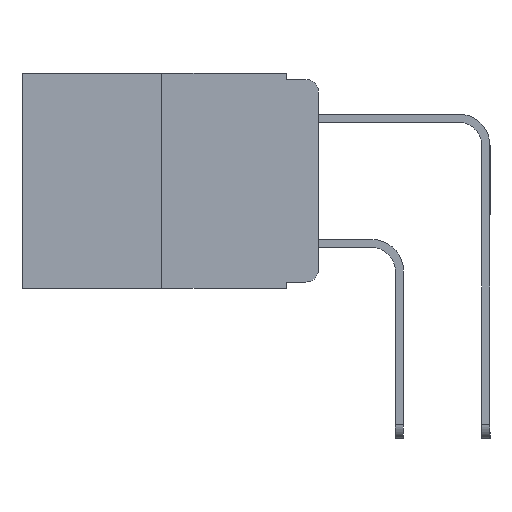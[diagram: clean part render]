
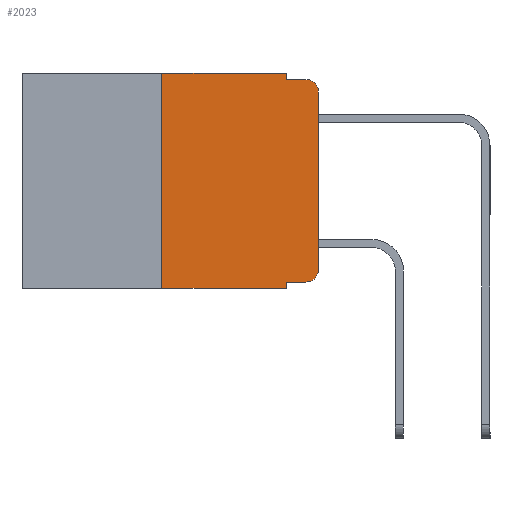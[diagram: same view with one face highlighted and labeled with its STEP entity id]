
A CAD part, left-side view. The second image highlights one B-rep face of the part: STEP entity #2023.
In plain terms, the highlighted planar face has unit normal (-1, 0, 0).
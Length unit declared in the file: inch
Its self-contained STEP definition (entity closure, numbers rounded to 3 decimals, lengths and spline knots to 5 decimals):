
#617 = LINE ( 'NONE', #1569, #8385 ) ;
#665 = LINE ( 'NONE', #15639, #1189 ) ;
#991 = ORIENTED_EDGE ( 'NONE', *, *, #13406, .F. ) ;
#1111 = VERTEX_POINT ( 'NONE', #16406 ) ;
#1169 = EDGE_CURVE ( 'NONE', #15016, #19149, #10449, .T. ) ;
#1189 = VECTOR ( 'NONE', #4652, 39.37008 ) ;
#1569 = CARTESIAN_POINT ( 'NONE',  ( 0., 0.25, 0. ) ) ;
#2023 = ADVANCED_FACE ( 'NONE', ( #3093 ), #8099, .F. ) ;
#2082 = VERTEX_POINT ( 'NONE', #9774 ) ;
#2101 = DIRECTION ( 'NONE',  ( 0., 0., -1. ) ) ;
#2270 = EDGE_CURVE ( 'NONE', #2365, #15016, #18591, .T. ) ;
#2335 = DIRECTION ( 'NONE',  ( -1., 0., 0. ) ) ;
#2365 = VERTEX_POINT ( 'NONE', #5889 ) ;
#3093 = FACE_OUTER_BOUND ( 'NONE', #9705, .T. ) ;
#3353 = ORIENTED_EDGE ( 'NONE', *, *, #5656, .F. ) ;
#3389 = EDGE_CURVE ( 'NONE', #2365, #6398, #12743, .T. ) ;
#3674 = LINE ( 'NONE', #16158, #15785 ) ;
#3875 = LINE ( 'NONE', #20039, #4422 ) ;
#3889 = CARTESIAN_POINT ( 'NONE',  ( 0., 0.051, -0.333 ) ) ;
#4422 = VECTOR ( 'NONE', #9297, 39.37008 ) ;
#4532 = EDGE_CURVE ( 'NONE', #1111, #14957, #617, .T. ) ;
#4652 = DIRECTION ( 'NONE',  ( 0., 0., -1. ) ) ;
#4967 = DIRECTION ( 'NONE',  ( -1., 0., 0. ) ) ;
#5305 = DIRECTION ( 'NONE',  ( 0., -1., 0. ) ) ;
#5582 = CARTESIAN_POINT ( 'NONE',  ( 0., 0.25, 0. ) ) ;
#5656 = EDGE_CURVE ( 'NONE', #16372, #13389, #665, .T. ) ;
#5866 = VERTEX_POINT ( 'NONE', #16166 ) ;
#5889 = CARTESIAN_POINT ( 'NONE',  ( 0., 0.051, -0.333 ) ) ;
#6398 = VERTEX_POINT ( 'NONE', #12817 ) ;
#6485 = CARTESIAN_POINT ( 'NONE',  ( 0., 0.473, 0. ) ) ;
#6742 = VECTOR ( 'NONE', #13379, 39.37008 ) ;
#7048 = ORIENTED_EDGE ( 'NONE', *, *, #2270, .T. ) ;
#7131 = ORIENTED_EDGE ( 'NONE', *, *, #9900, .T. ) ;
#7267 = ORIENTED_EDGE ( 'NONE', *, *, #18051, .T. ) ;
#7844 = EDGE_CURVE ( 'NONE', #13389, #5866, #14094, .T. ) ;
#7992 = CARTESIAN_POINT ( 'NONE',  ( 0., 0.473, -0.343 ) ) ;
#8065 = ORIENTED_EDGE ( 'NONE', *, *, #4532, .F. ) ;
#8099 = PLANE ( 'NONE',  #8270 ) ;
#8270 = AXIS2_PLACEMENT_3D ( 'NONE', #6485, #18849, #9643 ) ;
#8359 = ORIENTED_EDGE ( 'NONE', *, *, #8884, .T. ) ;
#8385 = VECTOR ( 'NONE', #20437, 39.37008 ) ;
#8790 = CIRCLE ( 'NONE', #16610, 0.02 ) ;
#8884 = EDGE_CURVE ( 'NONE', #2082, #5866, #8790, .T. ) ;
#9297 = DIRECTION ( 'NONE',  ( 0., 0., 1. ) ) ;
#9643 = DIRECTION ( 'NONE',  ( 0., 0., -1. ) ) ;
#9705 = EDGE_LOOP ( 'NONE', ( #7131, #8359, #18836, #3353, #991, #8065, #7267, #15604, #7048, #13803 ) ) ;
#9774 = CARTESIAN_POINT ( 'NONE',  ( 0., 0., -0.03 ) ) ;
#9900 = EDGE_CURVE ( 'NONE', #19149, #2082, #3875, .T. ) ;
#10092 = CARTESIAN_POINT ( 'NONE',  ( 0., 0.051, -0.01 ) ) ;
#10449 = CIRCLE ( 'NONE', #16633, 0.02 ) ;
#10468 = CARTESIAN_POINT ( 'NONE',  ( 0., 0.02, -0.333 ) ) ;
#11276 = VECTOR ( 'NONE', #17226, 39.37008 ) ;
#11700 = CARTESIAN_POINT ( 'NONE',  ( 0., 0.051, 0. ) ) ;
#11931 = CARTESIAN_POINT ( 'NONE',  ( 0., 0.02, -0.313 ) ) ;
#12255 = VECTOR ( 'NONE', #2101, 39.37008 ) ;
#12743 = LINE ( 'NONE', #11700, #12255 ) ;
#12817 = CARTESIAN_POINT ( 'NONE',  ( 0., 0.051, -0.343 ) ) ;
#13379 = DIRECTION ( 'NONE',  ( 0., -1., 0. ) ) ;
#13389 = VERTEX_POINT ( 'NONE', #10092 ) ;
#13406 = EDGE_CURVE ( 'NONE', #14957, #16372, #3674, .T. ) ;
#13506 = DIRECTION ( 'NONE',  ( 0., 0., -1. ) ) ;
#13803 = ORIENTED_EDGE ( 'NONE', *, *, #1169, .T. ) ;
#14094 = LINE ( 'NONE', #15061, #18660 ) ;
#14364 = CARTESIAN_POINT ( 'NONE',  ( 0., 0.02, -0.03 ) ) ;
#14430 = LINE ( 'NONE', #7992, #11276 ) ;
#14957 = VERTEX_POINT ( 'NONE', #5582 ) ;
#15016 = VERTEX_POINT ( 'NONE', #10468 ) ;
#15061 = CARTESIAN_POINT ( 'NONE',  ( 0., 0.051, -0.01 ) ) ;
#15461 = CARTESIAN_POINT ( 'NONE',  ( 0., 0., -0.313 ) ) ;
#15604 = ORIENTED_EDGE ( 'NONE', *, *, #3389, .F. ) ;
#15639 = CARTESIAN_POINT ( 'NONE',  ( 0., 0.051, 0. ) ) ;
#15785 = VECTOR ( 'NONE', #5305, 39.37008 ) ;
#15918 = DIRECTION ( 'NONE',  ( 0., 0., -1. ) ) ;
#16158 = CARTESIAN_POINT ( 'NONE',  ( 0., 0.473, 0. ) ) ;
#16166 = CARTESIAN_POINT ( 'NONE',  ( 0., 0.02, -0.01 ) ) ;
#16372 = VERTEX_POINT ( 'NONE', #17497 ) ;
#16406 = CARTESIAN_POINT ( 'NONE',  ( 0., 0.25, -0.343 ) ) ;
#16610 = AXIS2_PLACEMENT_3D ( 'NONE', #14364, #4967, #15918 ) ;
#16619 = DIRECTION ( 'NONE',  ( 0., -1., 0. ) ) ;
#16633 = AXIS2_PLACEMENT_3D ( 'NONE', #11931, #2335, #13506 ) ;
#17226 = DIRECTION ( 'NONE',  ( 0., -1., 0. ) ) ;
#17497 = CARTESIAN_POINT ( 'NONE',  ( 0., 0.051, 0. ) ) ;
#18051 = EDGE_CURVE ( 'NONE', #1111, #6398, #14430, .T. ) ;
#18591 = LINE ( 'NONE', #3889, #6742 ) ;
#18660 = VECTOR ( 'NONE', #16619, 39.37008 ) ;
#18836 = ORIENTED_EDGE ( 'NONE', *, *, #7844, .F. ) ;
#18849 = DIRECTION ( 'NONE',  ( 1., 0., 0. ) ) ;
#19149 = VERTEX_POINT ( 'NONE', #15461 ) ;
#20039 = CARTESIAN_POINT ( 'NONE',  ( 0., 0., 0. ) ) ;
#20437 = DIRECTION ( 'NONE',  ( 0., 0., 1. ) ) ;
